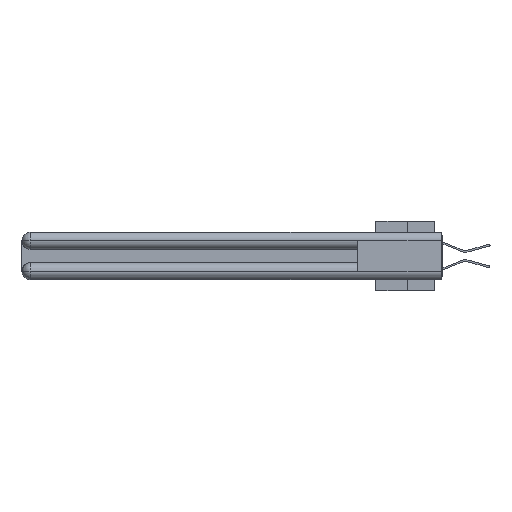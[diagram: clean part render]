
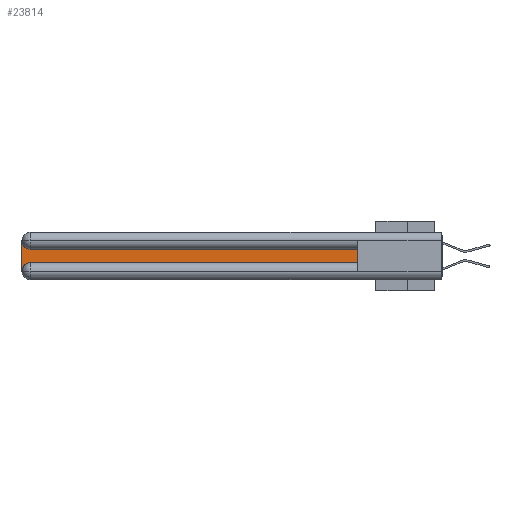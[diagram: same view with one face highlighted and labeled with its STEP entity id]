
A CAD part, left-side view. The second image highlights one B-rep face of the part: STEP entity #23814.
In plain terms, the highlighted planar face has unit normal (-1, 0, 0).
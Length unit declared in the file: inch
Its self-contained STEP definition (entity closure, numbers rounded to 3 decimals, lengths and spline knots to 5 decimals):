
#757 = EDGE_CURVE ( 'NONE', #12930, #18471, #17713, .T. ) ;
#1704 = FACE_OUTER_BOUND ( 'NONE', #30587, .T. ) ;
#2007 = CARTESIAN_POINT ( 'NONE',  ( 0.075, 0.6, -0.1225 ) ) ;
#3047 = EDGE_CURVE ( 'NONE', #23773, #6477, #25426, .T. ) ;
#3296 = CARTESIAN_POINT ( 'NONE',  ( 0.075, 2.94, -0.1225 ) ) ;
#3336 = VERTEX_POINT ( 'NONE', #3296 ) ;
#3771 = CARTESIAN_POINT ( 'NONE',  ( 0.075, 0.6, -0.2175 ) ) ;
#3929 = EDGE_CURVE ( 'NONE', #3336, #32614, #20863, .T. ) ;
#4852 = CARTESIAN_POINT ( 'NONE',  ( 0.075, 0.6, -0.2175 ) ) ;
#5683 = LINE ( 'NONE', #15773, #35243 ) ;
#5830 = ORIENTED_EDGE ( 'NONE', *, *, #8879, .T. ) ;
#6477 = VERTEX_POINT ( 'NONE', #14991 ) ;
#7013 = DIRECTION ( 'NONE',  ( 0., -1., 0. ) ) ;
#7976 = AXIS2_PLACEMENT_3D ( 'NONE', #9798, #21302, #24178 ) ;
#8879 = EDGE_CURVE ( 'NONE', #32614, #23773, #11169, .T. ) ;
#9798 = CARTESIAN_POINT ( 'NONE',  ( 0.075, 2.94, -0.0625 ) ) ;
#9944 = LINE ( 'NONE', #18577, #36780 ) ;
#11169 = LINE ( 'NONE', #30311, #24607 ) ;
#12930 = VERTEX_POINT ( 'NONE', #4852 ) ;
#14655 = DIRECTION ( 'NONE',  ( 0., 1., 0. ) ) ;
#14991 = CARTESIAN_POINT ( 'NONE',  ( 0.075, 2.94, -0.2175 ) ) ;
#15537 = ORIENTED_EDGE ( 'NONE', *, *, #3047, .T. ) ;
#15670 = EDGE_CURVE ( 'NONE', #6477, #12930, #5683, .T. ) ;
#15740 = CARTESIAN_POINT ( 'NONE',  ( 0.075, 3., -0.0625 ) ) ;
#15773 = CARTESIAN_POINT ( 'NONE',  ( 0.075, 0.6, -0.2175 ) ) ;
#17656 = DIRECTION ( 'NONE',  ( 1., 0., 0. ) ) ;
#17713 = LINE ( 'NONE', #3771, #29801 ) ;
#18457 = CARTESIAN_POINT ( 'NONE',  ( 0.075, 2.94, -0.2775 ) ) ;
#18471 = VERTEX_POINT ( 'NONE', #2007 ) ;
#18577 = CARTESIAN_POINT ( 'NONE',  ( 0.075, 0.6, -0.1225 ) ) ;
#20024 = PLANE ( 'NONE',  #27238 ) ;
#20143 = CARTESIAN_POINT ( 'NONE',  ( 0.075, 3., -0.1225 ) ) ;
#20527 = DIRECTION ( 'NONE',  ( 0., 0., -1. ) ) ;
#20863 = CIRCLE ( 'NONE', #7976, 0.06 ) ;
#21093 = AXIS2_PLACEMENT_3D ( 'NONE', #18457, #24219, #23847 ) ;
#21302 = DIRECTION ( 'NONE',  ( 1., 0., 0. ) ) ;
#21919 = ORIENTED_EDGE ( 'NONE', *, *, #757, .T. ) ;
#23773 = VERTEX_POINT ( 'NONE', #31824 ) ;
#23814 = ADVANCED_FACE ( 'NONE', ( #1704 ), #20024, .F. ) ;
#23847 = DIRECTION ( 'NONE',  ( 0., 0., -1. ) ) ;
#24178 = DIRECTION ( 'NONE',  ( 0., 0., -1. ) ) ;
#24219 = DIRECTION ( 'NONE',  ( 1., 0., 0. ) ) ;
#24607 = VECTOR ( 'NONE', #35531, 39.37008 ) ;
#25426 = CIRCLE ( 'NONE', #21093, 0.06 ) ;
#27188 = EDGE_CURVE ( 'NONE', #18471, #3336, #9944, .T. ) ;
#27238 = AXIS2_PLACEMENT_3D ( 'NONE', #20143, #17656, #20527 ) ;
#29294 = DIRECTION ( 'NONE',  ( 0., 0., 1. ) ) ;
#29801 = VECTOR ( 'NONE', #29294, 39.37008 ) ;
#30311 = CARTESIAN_POINT ( 'NONE',  ( 0.075, 3., -0.2175 ) ) ;
#30402 = ORIENTED_EDGE ( 'NONE', *, *, #27188, .T. ) ;
#30587 = EDGE_LOOP ( 'NONE', ( #30402, #35200, #5830, #15537, #31172, #21919 ) ) ;
#31172 = ORIENTED_EDGE ( 'NONE', *, *, #15670, .T. ) ;
#31824 = CARTESIAN_POINT ( 'NONE',  ( 0.075, 3., -0.2775 ) ) ;
#32614 = VERTEX_POINT ( 'NONE', #15740 ) ;
#35200 = ORIENTED_EDGE ( 'NONE', *, *, #3929, .T. ) ;
#35243 = VECTOR ( 'NONE', #7013, 39.37008 ) ;
#35531 = DIRECTION ( 'NONE',  ( 0., 0., -1. ) ) ;
#36780 = VECTOR ( 'NONE', #14655, 39.37008 ) ;
